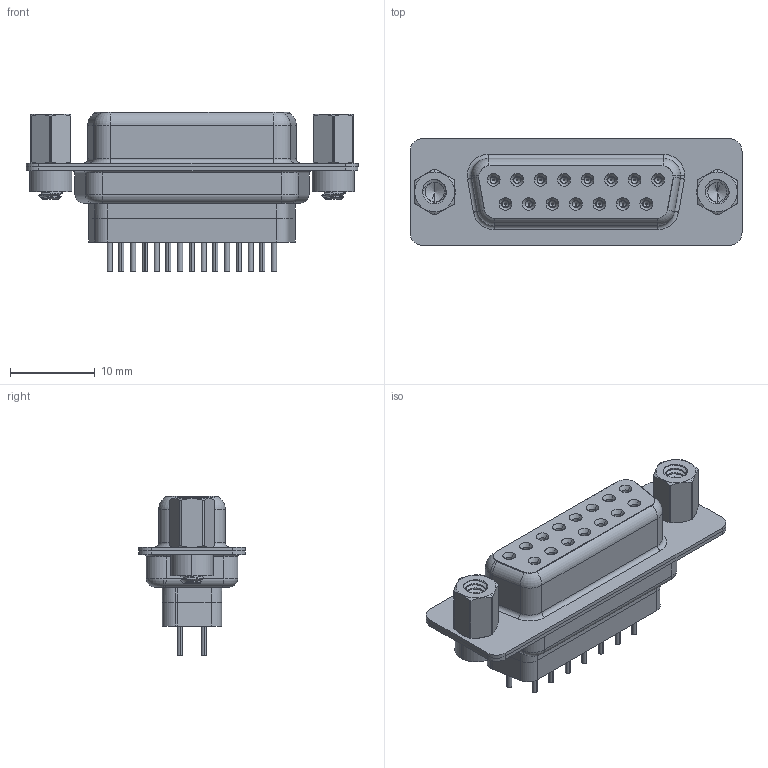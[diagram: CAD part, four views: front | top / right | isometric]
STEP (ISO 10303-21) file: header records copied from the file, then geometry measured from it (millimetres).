
FILE_DESCRIPTION (( 'STEP AP203' ), '1' );
FILE_NAME ('628-015-228-243.STEP', '2020-07-20T23:07:35', ( '' ), ( '' ), 'SwSTEP 2.0', 'SolidWorks 2020', '' );
FILE_SCHEMA (( 'CONFIG_CONTROL_DESIGN' ));
Length unit declared in the file: millimetre
Products named in the file (8): 628 4-40 Hex Standoff; 628-015-228-243; 628 Contact Row 1_28L; 628 Contact Row 2_28L; 628 Housing_15 FF; 628 Shell Rear_15 Contacts; 628 4-40 Threaded Rivet; 628 Shell Front_15 Contacts
Assembly tree (22 placements, depth 2):
  628-015-228-243
    628 Housing_15 FF
    628 Shell Front_15 Contacts
    628 Shell Rear_15 Contacts
    628 Contact Row 1_28L  x8
    628 Contact Row 2_28L  x7
    628 4-40 Threaded Rivet  x2
    628 4-40 Hex Standoff  x2
Bounding box: 39.15 x 12.6 x 18.8 mm (x, y, z)
Volume: 3123.9 mm3; surface area: 7508.5 mm2
Topology: 23 solids, 23 shells, 2347 faces, 5996 edges, 3736 vertices
Faces by surface type: cylinder 737, plane 560, torus 447, bspline 318, cone 285
Entity records: 29769 total; most frequent: CARTESIAN_POINT 10425, DIRECTION 3874, ORIENTED_EDGE 3776, EDGE_CURVE 1888, AXIS2_PLACEMENT_3D 1605, VERTEX_POINT 1193, EDGE_LOOP 897, CIRCLE 862
